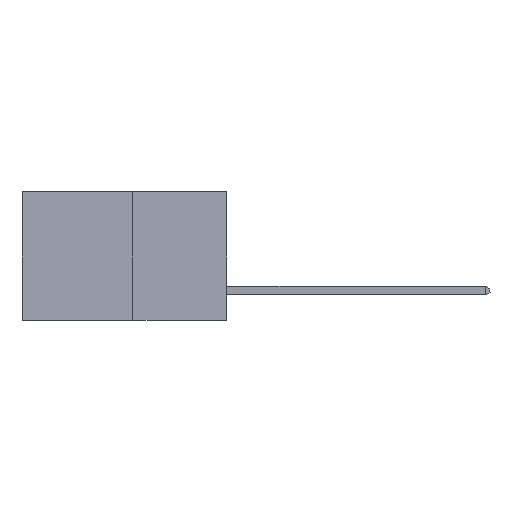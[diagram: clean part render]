
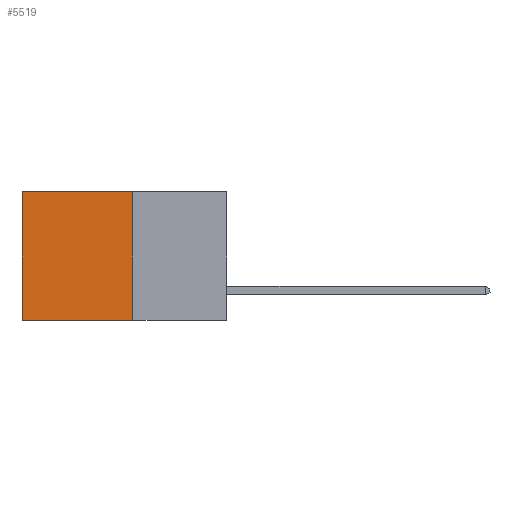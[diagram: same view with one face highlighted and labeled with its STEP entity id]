
A CAD part, left-side view. The second image highlights one B-rep face of the part: STEP entity #5519.
In plain terms, the highlighted planar face has unit normal (-1, 0, 0).
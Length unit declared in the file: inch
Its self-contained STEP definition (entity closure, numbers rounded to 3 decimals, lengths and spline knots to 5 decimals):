
#1691 = VECTOR ( 'NONE', #4777, 39.37008 ) ;
#2349 = CARTESIAN_POINT ( 'NONE',  ( 0.277, 0.27, -0.37 ) ) ;
#2778 = LINE ( 'NONE', #8736, #14486 ) ;
#4081 = CARTESIAN_POINT ( 'NONE',  ( 0.277, 0.27, -0.37 ) ) ;
#4777 = DIRECTION ( 'NONE',  ( 0., 1., 0. ) ) ;
#5519 = ADVANCED_FACE ( 'NONE', ( #27329 ), #28435, .F. ) ;
#8371 = ORIENTED_EDGE ( 'NONE', *, *, #29845, .T. ) ;
#8736 = CARTESIAN_POINT ( 'NONE',  ( 0.277, 0.59, -0.37 ) ) ;
#9047 = CARTESIAN_POINT ( 'NONE',  ( 0.277, 0.59, -0.37 ) ) ;
#10341 = ORIENTED_EDGE ( 'NONE', *, *, #22634, .F. ) ;
#11070 = DIRECTION ( 'NONE',  ( 0., 0., -1. ) ) ;
#12187 = LINE ( 'NONE', #22757, #23683 ) ;
#14486 = VECTOR ( 'NONE', #11070, 39.37008 ) ;
#15613 = ORIENTED_EDGE ( 'NONE', *, *, #18059, .F. ) ;
#15647 = CARTESIAN_POINT ( 'NONE',  ( 0.277, 0.27, -0.37 ) ) ;
#16775 = ORIENTED_EDGE ( 'NONE', *, *, #17058, .T. ) ;
#17058 = EDGE_CURVE ( 'NONE', #25952, #17445, #2778, .T. ) ;
#17445 = VERTEX_POINT ( 'NONE', #9047 ) ;
#17525 = CARTESIAN_POINT ( 'NONE',  ( 0.277, 0.59, 0. ) ) ;
#18059 = EDGE_CURVE ( 'NONE', #20776, #24654, #27772, .T. ) ;
#19031 = AXIS2_PLACEMENT_3D ( 'NONE', #28555, #25472, #25444 ) ;
#20216 = LINE ( 'NONE', #2349, #1691 ) ;
#20776 = VERTEX_POINT ( 'NONE', #26282 ) ;
#22634 = EDGE_CURVE ( 'NONE', #24654, #17445, #20216, .T. ) ;
#22757 = CARTESIAN_POINT ( 'NONE',  ( 0.277, 0.27, 0. ) ) ;
#23683 = VECTOR ( 'NONE', #25110, 39.37008 ) ;
#24398 = EDGE_LOOP ( 'NONE', ( #16775, #10341, #15613, #8371 ) ) ;
#24654 = VERTEX_POINT ( 'NONE', #15647 ) ;
#24828 = DIRECTION ( 'NONE',  ( 0., 0., -1. ) ) ;
#25110 = DIRECTION ( 'NONE',  ( 0., 1., 0. ) ) ;
#25444 = DIRECTION ( 'NONE',  ( 0., 0., -1. ) ) ;
#25472 = DIRECTION ( 'NONE',  ( 1., 0., 0. ) ) ;
#25952 = VERTEX_POINT ( 'NONE', #17525 ) ;
#26282 = CARTESIAN_POINT ( 'NONE',  ( 0.277, 0.27, 0. ) ) ;
#27329 = FACE_OUTER_BOUND ( 'NONE', #24398, .T. ) ;
#27772 = LINE ( 'NONE', #4081, #29240 ) ;
#28435 = PLANE ( 'NONE',  #19031 ) ;
#28555 = CARTESIAN_POINT ( 'NONE',  ( 0.277, 0.27, -0.37 ) ) ;
#29240 = VECTOR ( 'NONE', #24828, 39.37008 ) ;
#29845 = EDGE_CURVE ( 'NONE', #20776, #25952, #12187, .T. ) ;
